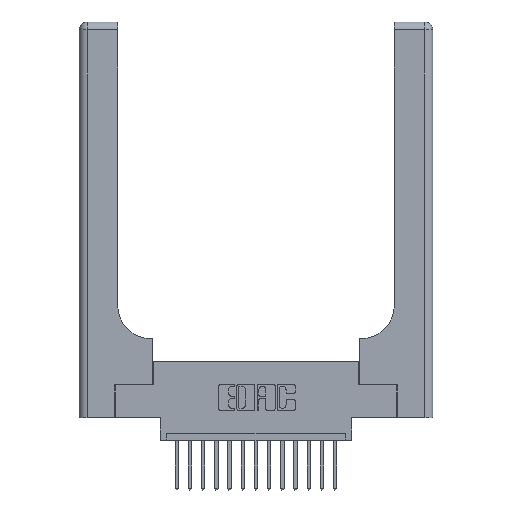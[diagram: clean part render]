
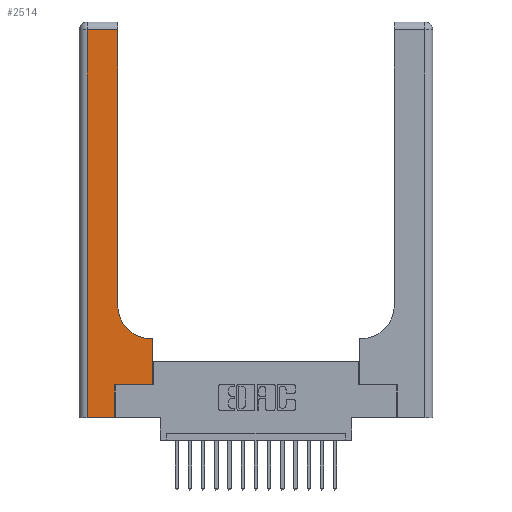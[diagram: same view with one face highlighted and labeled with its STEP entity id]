
A CAD part, top view. The second image highlights one B-rep face of the part: STEP entity #2514.
In plain terms, the highlighted planar face has unit normal (0, 0, 1).
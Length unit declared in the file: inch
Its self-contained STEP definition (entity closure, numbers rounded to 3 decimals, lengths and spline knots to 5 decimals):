
#427 = VERTEX_POINT ( 'NONE', #15599 ) ;
#776 = EDGE_CURVE ( 'NONE', #3438, #427, #8460, .T. ) ;
#1039 = ORIENTED_EDGE ( 'NONE', *, *, #4258, .T. ) ;
#1059 = EDGE_CURVE ( 'NONE', #5596, #8786, #1545, .T. ) ;
#1225 = AXIS2_PLACEMENT_3D ( 'NONE', #14571, #19006, #13248 ) ;
#1320 = VERTEX_POINT ( 'NONE', #14600 ) ;
#1527 = LINE ( 'NONE', #10633, #18023 ) ;
#1545 = LINE ( 'NONE', #5178, #1776 ) ;
#1748 = CARTESIAN_POINT ( 'NONE',  ( 0.2915, 2.94, 0.37 ) ) ;
#1776 = VECTOR ( 'NONE', #16864, 39.37008 ) ;
#1820 = EDGE_CURVE ( 'NONE', #427, #13970, #5647, .T. ) ;
#2304 = ORIENTED_EDGE ( 'NONE', *, *, #17529, .T. ) ;
#2514 = ADVANCED_FACE ( 'NONE', ( #9964 ), #7500, .F. ) ;
#2656 = VECTOR ( 'NONE', #18755, 39.37008 ) ;
#2744 = VERTEX_POINT ( 'NONE', #10573 ) ;
#2865 = ORIENTED_EDGE ( 'NONE', *, *, #7162, .T. ) ;
#3054 = VECTOR ( 'NONE', #9673, 39.37008 ) ;
#3398 = VECTOR ( 'NONE', #8402, 39.37008 ) ;
#3402 = ORIENTED_EDGE ( 'NONE', *, *, #13810, .T. ) ;
#3438 = VERTEX_POINT ( 'NONE', #10154 ) ;
#4083 = CARTESIAN_POINT ( 'NONE',  ( 0.269, 0., 0.37 ) ) ;
#4258 = EDGE_CURVE ( 'NONE', #8786, #3438, #14257, .T. ) ;
#4747 = CARTESIAN_POINT ( 'NONE',  ( 0., 3., 0.37 ) ) ;
#4913 = CARTESIAN_POINT ( 'NONE',  ( 0.5585, 0.25, 0.37 ) ) ;
#5178 = CARTESIAN_POINT ( 'NONE',  ( 0., 0., 0.37 ) ) ;
#5511 = CARTESIAN_POINT ( 'NONE',  ( 0.5585, 0.6, 0.37 ) ) ;
#5596 = VERTEX_POINT ( 'NONE', #18229 ) ;
#5647 = LINE ( 'NONE', #4913, #6808 ) ;
#5996 = VERTEX_POINT ( 'NONE', #1748 ) ;
#6799 = CARTESIAN_POINT ( 'NONE',  ( 0.269, 0.25, 0.37 ) ) ;
#6808 = VECTOR ( 'NONE', #15514, 39.37008 ) ;
#6895 = CARTESIAN_POINT ( 'NONE',  ( 0.2915, 3., 0.37 ) ) ;
#7162 = EDGE_CURVE ( 'NONE', #13970, #1320, #1527, .T. ) ;
#7500 = PLANE ( 'NONE',  #10302 ) ;
#8049 = DIRECTION ( 'NONE',  ( -1., 0., 0. ) ) ;
#8402 = DIRECTION ( 'NONE',  ( 1., 0., 0. ) ) ;
#8460 = LINE ( 'NONE', #6799, #3398 ) ;
#8786 = VERTEX_POINT ( 'NONE', #4083 ) ;
#8908 = ORIENTED_EDGE ( 'NONE', *, *, #18693, .T. ) ;
#9374 = EDGE_LOOP ( 'NONE', ( #8908, #3402, #2304, #14411, #1039, #13359, #17106, #2865, #18430 ) ) ;
#9648 = VECTOR ( 'NONE', #14868, 39.37008 ) ;
#9673 = DIRECTION ( 'NONE',  ( 0., 1., 0. ) ) ;
#9964 = FACE_OUTER_BOUND ( 'NONE', #9374, .T. ) ;
#10154 = CARTESIAN_POINT ( 'NONE',  ( 0.269, 0.25, 0.37 ) ) ;
#10302 = AXIS2_PLACEMENT_3D ( 'NONE', #4747, #12046, #14725 ) ;
#10573 = CARTESIAN_POINT ( 'NONE',  ( 0.06, 2.94, 0.37 ) ) ;
#10633 = CARTESIAN_POINT ( 'NONE',  ( 0.2915, 0.6, 0.37 ) ) ;
#12046 = DIRECTION ( 'NONE',  ( 0., 0., -1. ) ) ;
#12255 = LINE ( 'NONE', #6895, #18655 ) ;
#12611 = VERTEX_POINT ( 'NONE', #14135 ) ;
#13218 = EDGE_CURVE ( 'NONE', #1320, #12611, #17669, .T. ) ;
#13248 = DIRECTION ( 'NONE',  ( 1., 0., 0. ) ) ;
#13359 = ORIENTED_EDGE ( 'NONE', *, *, #776, .T. ) ;
#13810 = EDGE_CURVE ( 'NONE', #5996, #2744, #16261, .T. ) ;
#13970 = VERTEX_POINT ( 'NONE', #5511 ) ;
#14092 = LINE ( 'NONE', #17145, #2656 ) ;
#14135 = CARTESIAN_POINT ( 'NONE',  ( 0.2915, 0.85, 0.37 ) ) ;
#14257 = LINE ( 'NONE', #15486, #3054 ) ;
#14411 = ORIENTED_EDGE ( 'NONE', *, *, #1059, .T. ) ;
#14571 = CARTESIAN_POINT ( 'NONE',  ( 0.5415, 0.85, 0.37 ) ) ;
#14600 = CARTESIAN_POINT ( 'NONE',  ( 0.5415, 0.6, 0.37 ) ) ;
#14725 = DIRECTION ( 'NONE',  ( -1., 0., 0. ) ) ;
#14868 = DIRECTION ( 'NONE',  ( -1., 0., 0. ) ) ;
#15486 = CARTESIAN_POINT ( 'NONE',  ( 0.269, 0., 0.37 ) ) ;
#15514 = DIRECTION ( 'NONE',  ( 0., 1., 0. ) ) ;
#15599 = CARTESIAN_POINT ( 'NONE',  ( 0.5585, 0.25, 0.37 ) ) ;
#16261 = LINE ( 'NONE', #16928, #9648 ) ;
#16864 = DIRECTION ( 'NONE',  ( 1., 0., 0. ) ) ;
#16928 = CARTESIAN_POINT ( 'NONE',  ( 0., 2.94, 0.37 ) ) ;
#17105 = DIRECTION ( 'NONE',  ( 0., 1., 0. ) ) ;
#17106 = ORIENTED_EDGE ( 'NONE', *, *, #1820, .T. ) ;
#17145 = CARTESIAN_POINT ( 'NONE',  ( 0.06, 3., 0.37 ) ) ;
#17529 = EDGE_CURVE ( 'NONE', #2744, #5596, #14092, .T. ) ;
#17669 = CIRCLE ( 'NONE', #1225, 0.25 ) ;
#18023 = VECTOR ( 'NONE', #8049, 39.37008 ) ;
#18229 = CARTESIAN_POINT ( 'NONE',  ( 0.06, 0., 0.37 ) ) ;
#18430 = ORIENTED_EDGE ( 'NONE', *, *, #13218, .T. ) ;
#18655 = VECTOR ( 'NONE', #17105, 39.37008 ) ;
#18693 = EDGE_CURVE ( 'NONE', #12611, #5996, #12255, .T. ) ;
#18755 = DIRECTION ( 'NONE',  ( 0., -1., 0. ) ) ;
#19006 = DIRECTION ( 'NONE',  ( 0., 0., -1. ) ) ;
